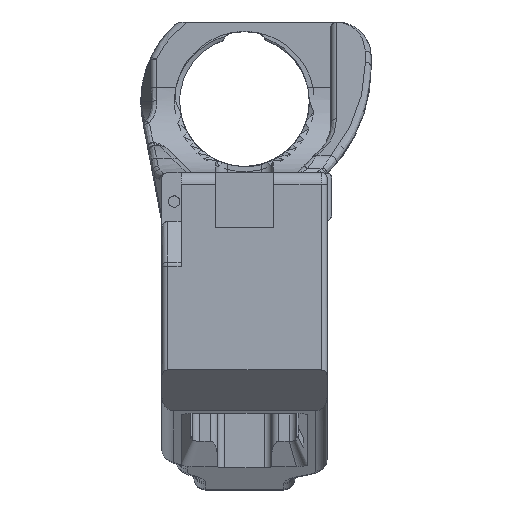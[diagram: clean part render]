
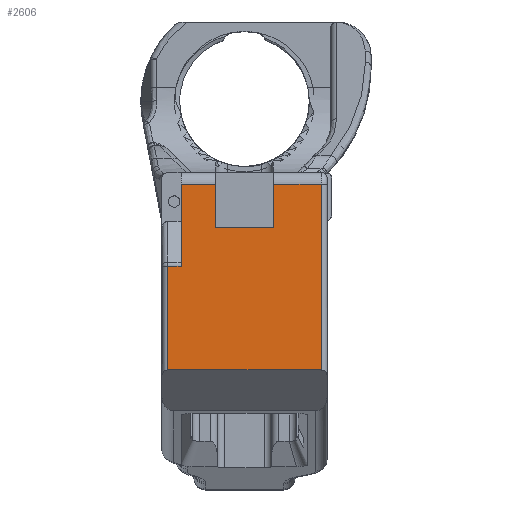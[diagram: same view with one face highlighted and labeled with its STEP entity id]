
A CAD part, top view. The second image highlights one B-rep face of the part: STEP entity #2606.
In plain terms, the highlighted planar face has unit normal (0, 0, 1).
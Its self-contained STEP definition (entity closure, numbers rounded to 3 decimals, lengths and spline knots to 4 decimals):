
#683 = CARTESIAN_POINT ( 'NONE',  ( 0.45, 0.15, 0.225 ) ) ;
#1064 = CARTESIAN_POINT ( 'NONE',  ( 0.3325, -0.5628, 0.225 ) ) ;
#1117 = CARTESIAN_POINT ( 'NONE',  ( 0.7475, -0.225, 0.225 ) ) ;
#1143 = CARTESIAN_POINT ( 'NONE',  ( 0.45, -0.5628, 0.225 ) ) ;
#1145 = CARTESIAN_POINT ( 'NONE',  ( 1.2525, -0.225, 0.225 ) ) ;
#1156 = CARTESIAN_POINT ( 'NONE',  ( 1.6675, -1.4638, 0.225 ) ) ;
#1198 = CARTESIAN_POINT ( 'NONE',  ( 1.6675, 0.15, 0.225 ) ) ;
#1939 = VERTEX_POINT ( 'NONE', #683 ) ;
#2323 = VERTEX_POINT ( 'NONE', #1064 ) ;
#2352 = VERTEX_POINT ( 'NONE', #1117 ) ;
#2366 = VERTEX_POINT ( 'NONE', #1143 ) ;
#2367 = VERTEX_POINT ( 'NONE', #1145 ) ;
#2373 = VERTEX_POINT ( 'NONE', #1156 ) ;
#2396 = VERTEX_POINT ( 'NONE', #1198 ) ;
#2606 = ADVANCED_FACE ( 'NONE', ( #37390 ), #37391, .F. ) ;
#8285 = CARTESIAN_POINT ( 'NONE',  ( 2., 0.15, 0.225 ) ) ;
#8290 = LINE ( 'NONE', #8285, #32780 ) ;
#8296 = DIRECTION ( 'NONE',  ( -1., 0., 0. ) ) ;
#9198 = AXIS2_PLACEMENT_3D ( 'NONE', #37387, #37394, #37395 ) ;
#9458 = EDGE_LOOP ( 'NONE', ( #31642, #31644, #31645, #31647, #31649, #31650, #31652, #31653, #31654, #31656 ) ) ;
#11581 = VERTEX_POINT ( 'NONE', #30760 ) ;
#14169 = CARTESIAN_POINT ( 'NONE',  ( 2.1, -1.4638, 0.225 ) ) ;
#14172 = LINE ( 'NONE', #14180, #33957 ) ;
#14173 = LINE ( 'NONE', #14183, #33959 ) ;
#14174 = LINE ( 'NONE', #14169, #33956 ) ;
#14178 = LINE ( 'NONE', #14185, #33960 ) ;
#14179 = DIRECTION ( 'NONE',  ( -1., 0., 0. ) ) ;
#14180 = CARTESIAN_POINT ( 'NONE',  ( 1.6675, 0.15, 0.225 ) ) ;
#14181 = LINE ( 'NONE', #14187, #33961 ) ;
#14182 = DIRECTION ( 'NONE',  ( 0., 1., 0. ) ) ;
#14183 = CARTESIAN_POINT ( 'NONE',  ( 1.2525, -0.225, 0.225 ) ) ;
#14184 = DIRECTION ( 'NONE',  ( 0., 1., 0. ) ) ;
#14185 = CARTESIAN_POINT ( 'NONE',  ( 0.7475, -0.225, 0.225 ) ) ;
#14186 = DIRECTION ( 'NONE',  ( 1., 0., 0. ) ) ;
#14187 = CARTESIAN_POINT ( 'NONE',  ( 0.7475, -0.225, 0.225 ) ) ;
#14188 = DIRECTION ( 'NONE',  ( 0., 1., 0. ) ) ;
#14189 = LINE ( 'NONE', #14190, #33963 ) ;
#14190 = CARTESIAN_POINT ( 'NONE',  ( 0.45, 0.25, 0.225 ) ) ;
#14191 = DIRECTION ( 'NONE',  ( 0., -1., 0. ) ) ;
#14192 = LINE ( 'NONE', #14193, #33964 ) ;
#14193 = CARTESIAN_POINT ( 'NONE',  ( 2., -0.5628, 0.225 ) ) ;
#14194 = DIRECTION ( 'NONE',  ( -1., 0., 0. ) ) ;
#14195 = LINE ( 'NONE', #14196, #33965 ) ;
#14196 = CARTESIAN_POINT ( 'NONE',  ( 0.3325, -1.4638, 0.225 ) ) ;
#14197 = DIRECTION ( 'NONE',  ( 0., -1., 0. ) ) ;
#16159 = CARTESIAN_POINT ( 'NONE',  ( 2., 0.15, 0.225 ) ) ;
#16161 = LINE ( 'NONE', #16159, #34180 ) ;
#16196 = DIRECTION ( 'NONE',  ( -1., 0., 0. ) ) ;
#16336 = CARTESIAN_POINT ( 'NONE',  ( 1.2525, 0.15, 0.225 ) ) ;
#16343 = CARTESIAN_POINT ( 'NONE',  ( 0.3325, -1.4638, 0.225 ) ) ;
#25637 = EDGE_CURVE ( 'NONE', #2373, #31989, #14174, .T. ) ;
#25638 = EDGE_CURVE ( 'NONE', #2373, #2396, #14172, .T. ) ;
#25639 = EDGE_CURVE ( 'NONE', #2367, #31982, #14173, .T. ) ;
#25640 = EDGE_CURVE ( 'NONE', #2352, #2367, #14178, .T. ) ;
#25641 = EDGE_CURVE ( 'NONE', #2352, #11581, #14181, .T. ) ;
#25642 = EDGE_CURVE ( 'NONE', #1939, #2366, #14189, .T. ) ;
#25643 = EDGE_CURVE ( 'NONE', #2366, #2323, #14192, .T. ) ;
#25644 = EDGE_CURVE ( 'NONE', #2323, #31989, #14195, .T. ) ;
#25978 = EDGE_CURVE ( 'NONE', #2396, #31982, #16161, .T. ) ;
#30760 = CARTESIAN_POINT ( 'NONE',  ( 0.7475, 0.15, 0.225 ) ) ;
#31642 = ORIENTED_EDGE ( 'NONE', *, *, #25637, .F. ) ;
#31644 = ORIENTED_EDGE ( 'NONE', *, *, #25638, .T. ) ;
#31645 = ORIENTED_EDGE ( 'NONE', *, *, #25978, .T. ) ;
#31647 = ORIENTED_EDGE ( 'NONE', *, *, #25639, .F. ) ;
#31649 = ORIENTED_EDGE ( 'NONE', *, *, #25640, .F. ) ;
#31650 = ORIENTED_EDGE ( 'NONE', *, *, #25641, .T. ) ;
#31652 = ORIENTED_EDGE ( 'NONE', *, *, #44715, .T. ) ;
#31653 = ORIENTED_EDGE ( 'NONE', *, *, #25642, .T. ) ;
#31654 = ORIENTED_EDGE ( 'NONE', *, *, #25643, .T. ) ;
#31656 = ORIENTED_EDGE ( 'NONE', *, *, #25644, .T. ) ;
#31982 = VERTEX_POINT ( 'NONE', #16336 ) ;
#31989 = VERTEX_POINT ( 'NONE', #16343 ) ;
#32780 = VECTOR ( 'NONE', #8296, 39.3701 ) ;
#33956 = VECTOR ( 'NONE', #14179, 39.3701 ) ;
#33957 = VECTOR ( 'NONE', #14182, 39.3701 ) ;
#33959 = VECTOR ( 'NONE', #14184, 39.3701 ) ;
#33960 = VECTOR ( 'NONE', #14186, 39.3701 ) ;
#33961 = VECTOR ( 'NONE', #14188, 39.3701 ) ;
#33963 = VECTOR ( 'NONE', #14191, 39.3701 ) ;
#33964 = VECTOR ( 'NONE', #14194, 39.3701 ) ;
#33965 = VECTOR ( 'NONE', #14197, 39.3701 ) ;
#34180 = VECTOR ( 'NONE', #16196, 39.3701 ) ;
#37387 = CARTESIAN_POINT ( 'NONE',  ( 2., -1.755, 0.225 ) ) ;
#37390 = FACE_OUTER_BOUND ( 'NONE', #9458, .T. ) ;
#37391 = PLANE ( 'NONE',  #9198 ) ;
#37394 = DIRECTION ( 'NONE',  ( 0., 0., -1. ) ) ;
#37395 = DIRECTION ( 'NONE',  ( 0., 1., 0. ) ) ;
#44715 = EDGE_CURVE ( 'NONE', #11581, #1939, #8290, .T. ) ;
